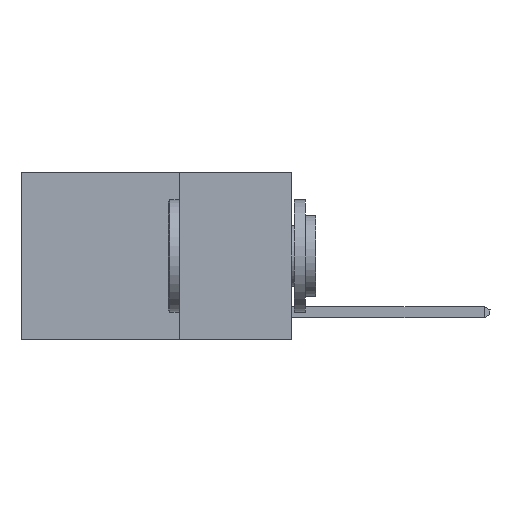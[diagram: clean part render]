
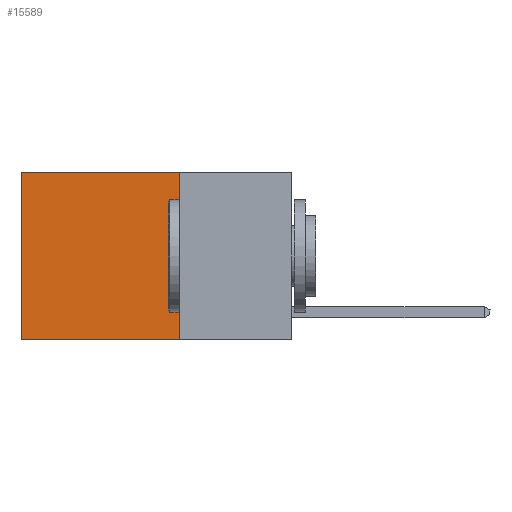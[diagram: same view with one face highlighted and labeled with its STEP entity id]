
A CAD part, left-side view. The second image highlights one B-rep face of the part: STEP entity #15589.
In plain terms, the highlighted planar face has unit normal (-1, 0, 0).
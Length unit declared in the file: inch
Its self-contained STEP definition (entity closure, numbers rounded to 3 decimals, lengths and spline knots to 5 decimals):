
#131 = EDGE_CURVE ( 'NONE', #12972, #3073, #8549, .T. ) ;
#553 = CARTESIAN_POINT ( 'NONE',  ( 0.2625, 0.25, -0.37 ) ) ;
#1191 = DIRECTION ( 'NONE',  ( 0., 1., 0. ) ) ;
#2218 = VECTOR ( 'NONE', #1191, 39.37008 ) ;
#2365 = DIRECTION ( 'NONE',  ( 0., 0., -1. ) ) ;
#2556 = VECTOR ( 'NONE', #15700, 39.37008 ) ;
#2630 = EDGE_LOOP ( 'NONE', ( #12148, #7502, #5063, #12170 ) ) ;
#2809 = CARTESIAN_POINT ( 'NONE',  ( 0.2625, 0.25, 0. ) ) ;
#3073 = VERTEX_POINT ( 'NONE', #7765 ) ;
#3405 = CARTESIAN_POINT ( 'NONE',  ( 0.2625, 0.6, 0. ) ) ;
#4425 = EDGE_CURVE ( 'NONE', #11359, #3073, #8782, .T. ) ;
#4675 = PLANE ( 'NONE',  #17930 ) ;
#5063 = ORIENTED_EDGE ( 'NONE', *, *, #13501, .F. ) ;
#5383 = VECTOR ( 'NONE', #2365, 39.37008 ) ;
#6013 = DIRECTION ( 'NONE',  ( 0., 0., -1. ) ) ;
#7502 = ORIENTED_EDGE ( 'NONE', *, *, #4425, .F. ) ;
#7765 = CARTESIAN_POINT ( 'NONE',  ( 0.2625, 0.6, -0.37 ) ) ;
#8465 = CARTESIAN_POINT ( 'NONE',  ( 0.2625, 0.6, 0. ) ) ;
#8549 = LINE ( 'NONE', #8465, #9591 ) ;
#8782 = LINE ( 'NONE', #553, #2556 ) ;
#9374 = CARTESIAN_POINT ( 'NONE',  ( 0.2625, 0.25, -0.37 ) ) ;
#9591 = VECTOR ( 'NONE', #6013, 39.37008 ) ;
#11359 = VERTEX_POINT ( 'NONE', #9374 ) ;
#11579 = DIRECTION ( 'NONE',  ( 1., 0., 0. ) ) ;
#11663 = DIRECTION ( 'NONE',  ( 0., 0., -1. ) ) ;
#11888 = CARTESIAN_POINT ( 'NONE',  ( 0.2625, 0.25, 0. ) ) ;
#12148 = ORIENTED_EDGE ( 'NONE', *, *, #131, .T. ) ;
#12170 = ORIENTED_EDGE ( 'NONE', *, *, #12298, .T. ) ;
#12298 = EDGE_CURVE ( 'NONE', #14596, #12972, #15311, .T. ) ;
#12972 = VERTEX_POINT ( 'NONE', #3405 ) ;
#13501 = EDGE_CURVE ( 'NONE', #14596, #11359, #16350, .T. ) ;
#14596 = VERTEX_POINT ( 'NONE', #16385 ) ;
#15311 = LINE ( 'NONE', #2809, #2218 ) ;
#15589 = ADVANCED_FACE ( 'NONE', ( #17300 ), #4675, .F. ) ;
#15700 = DIRECTION ( 'NONE',  ( 0., 1., 0. ) ) ;
#15937 = CARTESIAN_POINT ( 'NONE',  ( 0.2625, 0.25, 0. ) ) ;
#16350 = LINE ( 'NONE', #11888, #5383 ) ;
#16385 = CARTESIAN_POINT ( 'NONE',  ( 0.2625, 0.25, 0. ) ) ;
#17300 = FACE_OUTER_BOUND ( 'NONE', #2630, .T. ) ;
#17930 = AXIS2_PLACEMENT_3D ( 'NONE', #15937, #11579, #11663 ) ;
